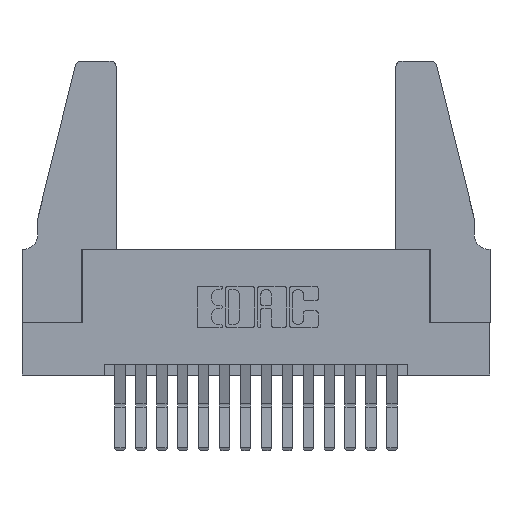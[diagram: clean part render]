
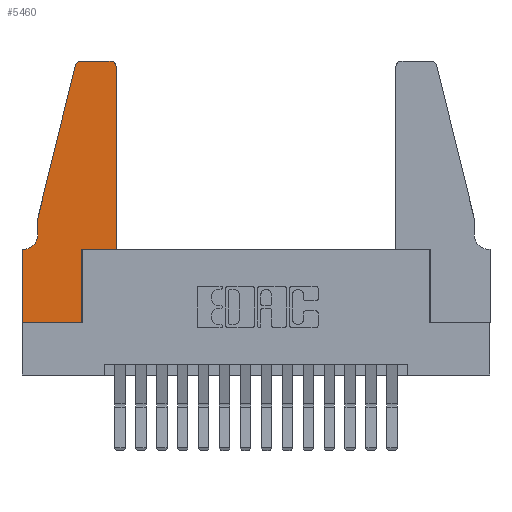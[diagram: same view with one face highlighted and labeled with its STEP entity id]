
A CAD part, top view. The second image highlights one B-rep face of the part: STEP entity #5460.
In plain terms, the highlighted planar face has unit normal (0, 0, 1).
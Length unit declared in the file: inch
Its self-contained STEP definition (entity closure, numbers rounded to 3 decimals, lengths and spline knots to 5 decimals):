
#153 = VERTEX_POINT ( 'NONE', #1888 ) ;
#297 = EDGE_CURVE ( 'NONE', #2057, #8815, #3517, .T. ) ;
#370 = DIRECTION ( 'NONE',  ( 1., 0., 0. ) ) ;
#597 = DIRECTION ( 'NONE',  ( 0., 0., 1. ) ) ;
#1093 = DIRECTION ( 'NONE',  ( 0., 0., 1. ) ) ;
#1131 = VERTEX_POINT ( 'NONE', #15465 ) ;
#1138 = LINE ( 'NONE', #11803, #6085 ) ;
#1187 = ORIENTED_EDGE ( 'NONE', *, *, #9265, .T. ) ;
#1389 = LINE ( 'NONE', #4440, #11083 ) ;
#1442 = EDGE_CURVE ( 'NONE', #11162, #1131, #2886, .T. ) ;
#1546 = DIRECTION ( 'NONE',  ( -0.239, -0.971, 0. ) ) ;
#1554 = ORIENTED_EDGE ( 'NONE', *, *, #9931, .T. ) ;
#1592 = CARTESIAN_POINT ( 'NONE',  ( 0., 0., 0.37 ) ) ;
#1811 = ORIENTED_EDGE ( 'NONE', *, *, #1442, .T. ) ;
#1888 = CARTESIAN_POINT ( 'NONE',  ( 0.4205, 1.25, 0.37 ) ) ;
#2057 = VERTEX_POINT ( 'NONE', #1592 ) ;
#2191 = CARTESIAN_POINT ( 'NONE',  ( 0.4505, 0.35, 0.37 ) ) ;
#2201 = CIRCLE ( 'NONE', #6767, 0.07 ) ;
#2730 = VERTEX_POINT ( 'NONE', #3989 ) ;
#2837 = ORIENTED_EDGE ( 'NONE', *, *, #4080, .T. ) ;
#2886 = LINE ( 'NONE', #9648, #6587 ) ;
#3070 = EDGE_CURVE ( 'NONE', #12710, #2057, #1389, .T. ) ;
#3494 = VERTEX_POINT ( 'NONE', #6175 ) ;
#3517 = LINE ( 'NONE', #13887, #10527 ) ;
#3528 = EDGE_CURVE ( 'NONE', #153, #10504, #11892, .T. ) ;
#3600 = CARTESIAN_POINT ( 'NONE',  ( 0.2605, 1.25, 0.37 ) ) ;
#3989 = CARTESIAN_POINT ( 'NONE',  ( 0.2865, 0.35, 0.37 ) ) ;
#4080 = EDGE_CURVE ( 'NONE', #6594, #11162, #7516, .T. ) ;
#4257 = CARTESIAN_POINT ( 'NONE',  ( 0.284, 1.22, 0.37 ) ) ;
#4440 = CARTESIAN_POINT ( 'NONE',  ( 0., 0., 0.37 ) ) ;
#4470 = DIRECTION ( 'NONE',  ( -1., 0., 0. ) ) ;
#4743 = ORIENTED_EDGE ( 'NONE', *, *, #297, .T. ) ;
#4809 = ORIENTED_EDGE ( 'NONE', *, *, #8853, .T. ) ;
#5460 = ADVANCED_FACE ( 'NONE', ( #13849 ), #8297, .T. ) ;
#5577 = DIRECTION ( 'NONE',  ( 1., 0., 0. ) ) ;
#5719 = VERTEX_POINT ( 'NONE', #11300 ) ;
#5787 = CARTESIAN_POINT ( 'NONE',  ( 0.0055, 0.42, 0.37 ) ) ;
#5862 = CIRCLE ( 'NONE', #9337, 0.03 ) ;
#6085 = VECTOR ( 'NONE', #14369, 39.37008 ) ;
#6089 = AXIS2_PLACEMENT_3D ( 'NONE', #6921, #597, #370 ) ;
#6175 = CARTESIAN_POINT ( 'NONE',  ( 0.0055, 0.35, 0.37 ) ) ;
#6408 = EDGE_CURVE ( 'NONE', #10837, #5719, #12573, .T. ) ;
#6466 = LINE ( 'NONE', #9445, #7907 ) ;
#6587 = VECTOR ( 'NONE', #14875, 39.37008 ) ;
#6594 = VERTEX_POINT ( 'NONE', #11051 ) ;
#6659 = ORIENTED_EDGE ( 'NONE', *, *, #6408, .T. ) ;
#6767 = AXIS2_PLACEMENT_3D ( 'NONE', #5787, #12349, #4470 ) ;
#6921 = CARTESIAN_POINT ( 'NONE',  ( 0., 0.35, 0.37 ) ) ;
#7472 = CARTESIAN_POINT ( 'NONE',  ( 0.4205, 1.22, 0.37 ) ) ;
#7516 = LINE ( 'NONE', #15236, #8119 ) ;
#7907 = VECTOR ( 'NONE', #12157, 39.37008 ) ;
#8119 = VECTOR ( 'NONE', #1546, 39.37008 ) ;
#8297 = PLANE ( 'NONE',  #6089 ) ;
#8815 = VERTEX_POINT ( 'NONE', #9920 ) ;
#8853 = EDGE_CURVE ( 'NONE', #1131, #3494, #2201, .T. ) ;
#9143 = ORIENTED_EDGE ( 'NONE', *, *, #3070, .T. ) ;
#9265 = EDGE_CURVE ( 'NONE', #2730, #10837, #10205, .T. ) ;
#9283 = CIRCLE ( 'NONE', #12669, 0.03 ) ;
#9337 = AXIS2_PLACEMENT_3D ( 'NONE', #7472, #1093, #15578 ) ;
#9445 = CARTESIAN_POINT ( 'NONE',  ( 0.2865, 0.35, 0.37 ) ) ;
#9496 = ORIENTED_EDGE ( 'NONE', *, *, #16228, .T. ) ;
#9519 = EDGE_CURVE ( 'NONE', #8815, #2730, #6466, .T. ) ;
#9576 = VECTOR ( 'NONE', #9956, 39.37008 ) ;
#9648 = CARTESIAN_POINT ( 'NONE',  ( 0.0755, 0.5, 0.37 ) ) ;
#9920 = CARTESIAN_POINT ( 'NONE',  ( 0.2865, 0., 0.37 ) ) ;
#9931 = EDGE_CURVE ( 'NONE', #5719, #153, #5862, .T. ) ;
#9956 = DIRECTION ( 'NONE',  ( 1., 0., 0. ) ) ;
#10205 = LINE ( 'NONE', #2191, #9576 ) ;
#10504 = VERTEX_POINT ( 'NONE', #15531 ) ;
#10527 = VECTOR ( 'NONE', #16462, 39.37008 ) ;
#10746 = ORIENTED_EDGE ( 'NONE', *, *, #12229, .T. ) ;
#10837 = VERTEX_POINT ( 'NONE', #12765 ) ;
#11051 = CARTESIAN_POINT ( 'NONE',  ( 0.25487, 1.22718, 0.37 ) ) ;
#11083 = VECTOR ( 'NONE', #14938, 39.37008 ) ;
#11162 = VERTEX_POINT ( 'NONE', #16177 ) ;
#11300 = CARTESIAN_POINT ( 'NONE',  ( 0.4505, 1.22, 0.37 ) ) ;
#11803 = CARTESIAN_POINT ( 'NONE',  ( 0.0755, 0.35, 0.37 ) ) ;
#11892 = LINE ( 'NONE', #3600, #13931 ) ;
#12157 = DIRECTION ( 'NONE',  ( 0., 1., 0. ) ) ;
#12229 = EDGE_CURVE ( 'NONE', #10504, #6594, #9283, .T. ) ;
#12262 = ORIENTED_EDGE ( 'NONE', *, *, #3528, .T. ) ;
#12349 = DIRECTION ( 'NONE',  ( 0., 0., -1. ) ) ;
#12573 = LINE ( 'NONE', #16874, #15223 ) ;
#12635 = ORIENTED_EDGE ( 'NONE', *, *, #9519, .T. ) ;
#12669 = AXIS2_PLACEMENT_3D ( 'NONE', #4257, #13445, #5577 ) ;
#12710 = VERTEX_POINT ( 'NONE', #16050 ) ;
#12765 = CARTESIAN_POINT ( 'NONE',  ( 0.4505, 0.35, 0.37 ) ) ;
#13445 = DIRECTION ( 'NONE',  ( 0., 0., 1. ) ) ;
#13849 = FACE_OUTER_BOUND ( 'NONE', #14194, .T. ) ;
#13887 = CARTESIAN_POINT ( 'NONE',  ( 0., 0., 0.37 ) ) ;
#13931 = VECTOR ( 'NONE', #14110, 39.37008 ) ;
#14110 = DIRECTION ( 'NONE',  ( -1., 0., 0. ) ) ;
#14194 = EDGE_LOOP ( 'NONE', ( #12262, #10746, #2837, #1811, #4809, #9496, #9143, #4743, #12635, #1187, #6659, #1554 ) ) ;
#14369 = DIRECTION ( 'NONE',  ( -1., 0., 0. ) ) ;
#14875 = DIRECTION ( 'NONE',  ( 0., -1., 0. ) ) ;
#14938 = DIRECTION ( 'NONE',  ( 0., -1., 0. ) ) ;
#15223 = VECTOR ( 'NONE', #15620, 39.37008 ) ;
#15236 = CARTESIAN_POINT ( 'NONE',  ( 0.0755, 0.5, 0.37 ) ) ;
#15465 = CARTESIAN_POINT ( 'NONE',  ( 0.0755, 0.42, 0.37 ) ) ;
#15531 = CARTESIAN_POINT ( 'NONE',  ( 0.284, 1.25, 0.37 ) ) ;
#15578 = DIRECTION ( 'NONE',  ( 1., 0., 0. ) ) ;
#15620 = DIRECTION ( 'NONE',  ( 0., 1., 0. ) ) ;
#16050 = CARTESIAN_POINT ( 'NONE',  ( 0., 0.35, 0.37 ) ) ;
#16177 = CARTESIAN_POINT ( 'NONE',  ( 0.0755, 0.5, 0.37 ) ) ;
#16228 = EDGE_CURVE ( 'NONE', #3494, #12710, #1138, .T. ) ;
#16462 = DIRECTION ( 'NONE',  ( 1., 0., 0. ) ) ;
#16874 = CARTESIAN_POINT ( 'NONE',  ( 0.4505, 0.35, 0.37 ) ) ;
